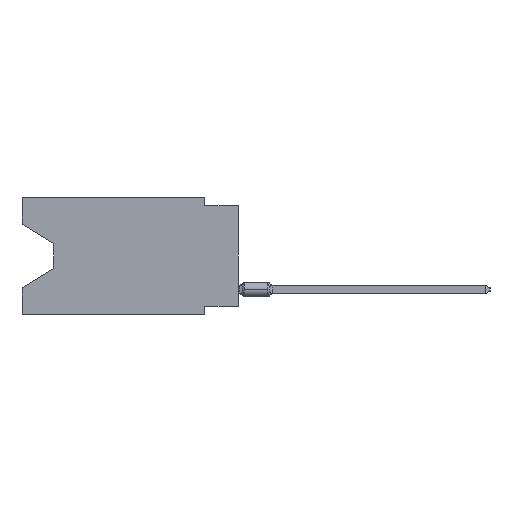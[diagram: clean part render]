
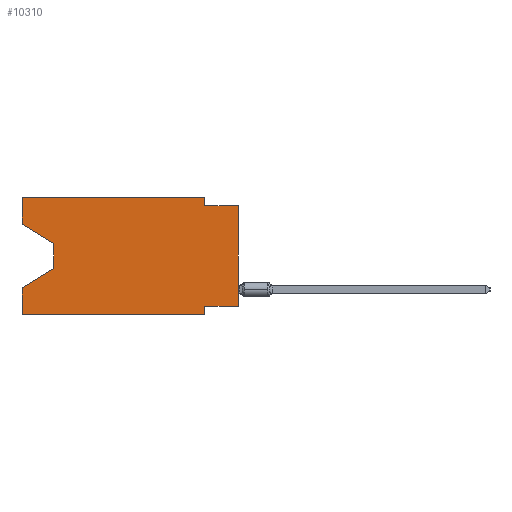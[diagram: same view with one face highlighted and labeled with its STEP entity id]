
A CAD part, left-side view. The second image highlights one B-rep face of the part: STEP entity #10310.
In plain terms, the highlighted planar face has unit normal (-1, 0, 0).
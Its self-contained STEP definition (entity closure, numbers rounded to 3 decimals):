
#645 = EDGE_CURVE ( 'NONE', #43866, #42756, #50582, .T. ) ;
#1397 = DIRECTION ( 'NONE',  ( 0., -1., 0. ) ) ;
#1641 = CARTESIAN_POINT ( 'NONE',  ( 0., 0., -0.635 ) ) ;
#1836 = CARTESIAN_POINT ( 'NONE',  ( 0., 16.383, -2.038 ) ) ;
#3748 = CARTESIAN_POINT ( 'NONE',  ( 0., 16.383, -6.852 ) ) ;
#4718 = EDGE_CURVE ( 'NONE', #44274, #43866, #31832, .T. ) ;
#5734 = ORIENTED_EDGE ( 'NONE', *, *, #28467, .F. ) ;
#6387 = DIRECTION ( 'NONE',  ( 0., 0., -1. ) ) ;
#6428 = DIRECTION ( 'NONE',  ( 0., 0., 1. ) ) ;
#6857 = CARTESIAN_POINT ( 'NONE',  ( 0., 16.383, 0. ) ) ;
#7142 = PLANE ( 'NONE',  #22139 ) ;
#7322 = VECTOR ( 'NONE', #1397, 1000. ) ;
#7587 = CARTESIAN_POINT ( 'NONE',  ( 0., 16.383, 0. ) ) ;
#8162 = DIRECTION ( 'NONE',  ( 0., -1., 0. ) ) ;
#8312 = VERTEX_POINT ( 'NONE', #28865 ) ;
#8632 = ORIENTED_EDGE ( 'NONE', *, *, #11054, .F. ) ;
#8651 = CARTESIAN_POINT ( 'NONE',  ( 0., 0., -8.255 ) ) ;
#9050 = VECTOR ( 'NONE', #55204, 1000. ) ;
#10310 = ADVANCED_FACE ( 'NONE', ( #44839 ), #7142, .F. ) ;
#10896 = LINE ( 'NONE', #27638, #35530 ) ;
#11054 = EDGE_CURVE ( 'NONE', #16255, #39012, #20406, .T. ) ;
#12053 = ORIENTED_EDGE ( 'NONE', *, *, #40500, .F. ) ;
#12149 = VERTEX_POINT ( 'NONE', #8651 ) ;
#12476 = CARTESIAN_POINT ( 'NONE',  ( 0., 2.54, -8.89 ) ) ;
#12739 = LINE ( 'NONE', #54389, #34710 ) ;
#13559 = VERTEX_POINT ( 'NONE', #53108 ) ;
#13908 = CARTESIAN_POINT ( 'NONE',  ( 0., 13.97, -5.385 ) ) ;
#14532 = LINE ( 'NONE', #27086, #7322 ) ;
#16251 = CARTESIAN_POINT ( 'NONE',  ( 0., 0., -0.635 ) ) ;
#16255 = VERTEX_POINT ( 'NONE', #1836 ) ;
#16751 = EDGE_CURVE ( 'NONE', #13559, #47408, #53030, .T. ) ;
#17065 = ORIENTED_EDGE ( 'NONE', *, *, #51030, .F. ) ;
#20304 = VECTOR ( 'NONE', #45476, 1000. ) ;
#20406 = LINE ( 'NONE', #40805, #43593 ) ;
#21121 = CARTESIAN_POINT ( 'NONE',  ( 0., 16.383, -2.038 ) ) ;
#21954 = CARTESIAN_POINT ( 'NONE',  ( 0., 13.97, -3.505 ) ) ;
#22120 = VERTEX_POINT ( 'NONE', #1641 ) ;
#22139 = AXIS2_PLACEMENT_3D ( 'NONE', #6857, #23890, #32248 ) ;
#23890 = DIRECTION ( 'NONE',  ( 1., 0., 0. ) ) ;
#24862 = DIRECTION ( 'NONE',  ( 0., 0., 1. ) ) ;
#24960 = ORIENTED_EDGE ( 'NONE', *, *, #4718, .T. ) ;
#26167 = ORIENTED_EDGE ( 'NONE', *, *, #53547, .T. ) ;
#27086 = CARTESIAN_POINT ( 'NONE',  ( 0., 16.383, -8.89 ) ) ;
#27532 = ORIENTED_EDGE ( 'NONE', *, *, #645, .T. ) ;
#27638 = CARTESIAN_POINT ( 'NONE',  ( 0., 16.383, 0. ) ) ;
#27923 = DIRECTION ( 'NONE',  ( 0., 0., -1. ) ) ;
#28238 = VECTOR ( 'NONE', #42479, 1000. ) ;
#28467 = EDGE_CURVE ( 'NONE', #12149, #8312, #35781, .T. ) ;
#28865 = CARTESIAN_POINT ( 'NONE',  ( 0., 2.54, -8.255 ) ) ;
#29531 = VERTEX_POINT ( 'NONE', #29854 ) ;
#29760 = DIRECTION ( 'NONE',  ( 0., 0., 1. ) ) ;
#29854 = CARTESIAN_POINT ( 'NONE',  ( 0., 16.383, -8.89 ) ) ;
#30310 = VECTOR ( 'NONE', #39171, 1000. ) ;
#31832 = LINE ( 'NONE', #53087, #33377 ) ;
#32111 = CARTESIAN_POINT ( 'NONE',  ( 0., 16.383, 0. ) ) ;
#32248 = DIRECTION ( 'NONE',  ( 0., 0., -1. ) ) ;
#32341 = EDGE_CURVE ( 'NONE', #8312, #47525, #37637, .T. ) ;
#33377 = VECTOR ( 'NONE', #27923, 1000. ) ;
#34710 = VECTOR ( 'NONE', #29760, 1000. ) ;
#35530 = VECTOR ( 'NONE', #6428, 1000. ) ;
#35781 = LINE ( 'NONE', #53103, #30310 ) ;
#35970 = ORIENTED_EDGE ( 'NONE', *, *, #16751, .F. ) ;
#36538 = CARTESIAN_POINT ( 'NONE',  ( 0., 2.54, -8.89 ) ) ;
#37165 = EDGE_CURVE ( 'NONE', #29531, #47525, #14532, .T. ) ;
#37637 = LINE ( 'NONE', #36538, #20304 ) ;
#37866 = LINE ( 'NONE', #21121, #9050 ) ;
#39012 = VERTEX_POINT ( 'NONE', #7587 ) ;
#39171 = DIRECTION ( 'NONE',  ( 0., 1., 0. ) ) ;
#39658 = VECTOR ( 'NONE', #48613, 1000. ) ;
#39964 = LINE ( 'NONE', #32111, #39658 ) ;
#40500 = EDGE_CURVE ( 'NONE', #39012, #13559, #39964, .T. ) ;
#40805 = CARTESIAN_POINT ( 'NONE',  ( 0., 16.383, 0. ) ) ;
#40991 = CARTESIAN_POINT ( 'NONE',  ( 0., 2.54, -0.635 ) ) ;
#42479 = DIRECTION ( 'NONE',  ( 0., 0.855, -0.519 ) ) ;
#42756 = VERTEX_POINT ( 'NONE', #3748 ) ;
#43447 = ORIENTED_EDGE ( 'NONE', *, *, #46332, .T. ) ;
#43593 = VECTOR ( 'NONE', #24862, 1000. ) ;
#43643 = ORIENTED_EDGE ( 'NONE', *, *, #32341, .F. ) ;
#43866 = VERTEX_POINT ( 'NONE', #13908 ) ;
#44274 = VERTEX_POINT ( 'NONE', #21954 ) ;
#44658 = CARTESIAN_POINT ( 'NONE',  ( 0., 2.54, 0. ) ) ;
#44717 = ORIENTED_EDGE ( 'NONE', *, *, #45769, .F. ) ;
#44839 = FACE_OUTER_BOUND ( 'NONE', #52125, .T. ) ;
#45476 = DIRECTION ( 'NONE',  ( 0., 0., -1. ) ) ;
#45769 = EDGE_CURVE ( 'NONE', #29531, #42756, #10896, .T. ) ;
#45826 = VECTOR ( 'NONE', #6387, 1000. ) ;
#46101 = ORIENTED_EDGE ( 'NONE', *, *, #37165, .T. ) ;
#46332 = EDGE_CURVE ( 'NONE', #12149, #22120, #12739, .T. ) ;
#46412 = CARTESIAN_POINT ( 'NONE',  ( 0., 13.97, -5.385 ) ) ;
#47237 = VECTOR ( 'NONE', #8162, 1000. ) ;
#47408 = VERTEX_POINT ( 'NONE', #40991 ) ;
#47525 = VERTEX_POINT ( 'NONE', #12476 ) ;
#48613 = DIRECTION ( 'NONE',  ( 0., -1., 0. ) ) ;
#50582 = LINE ( 'NONE', #46412, #28238 ) ;
#51030 = EDGE_CURVE ( 'NONE', #47408, #22120, #53959, .T. ) ;
#52125 = EDGE_LOOP ( 'NONE', ( #26167, #24960, #27532, #44717, #46101, #43643, #5734, #43447, #17065, #35970, #12053, #8632 ) ) ;
#53030 = LINE ( 'NONE', #44658, #45826 ) ;
#53087 = CARTESIAN_POINT ( 'NONE',  ( 0., 13.97, -3.505 ) ) ;
#53103 = CARTESIAN_POINT ( 'NONE',  ( 0., 0., -8.255 ) ) ;
#53108 = CARTESIAN_POINT ( 'NONE',  ( 0., 2.54, 0. ) ) ;
#53547 = EDGE_CURVE ( 'NONE', #16255, #44274, #37866, .T. ) ;
#53959 = LINE ( 'NONE', #16251, #47237 ) ;
#54389 = CARTESIAN_POINT ( 'NONE',  ( 0., 0., 0. ) ) ;
#55204 = DIRECTION ( 'NONE',  ( 0., -0.855, -0.519 ) ) ;
